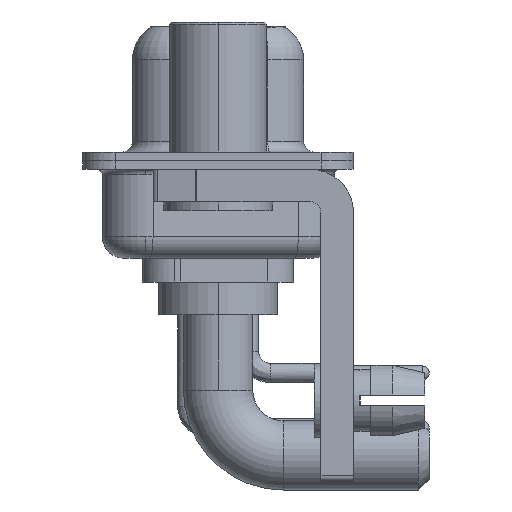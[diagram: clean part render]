
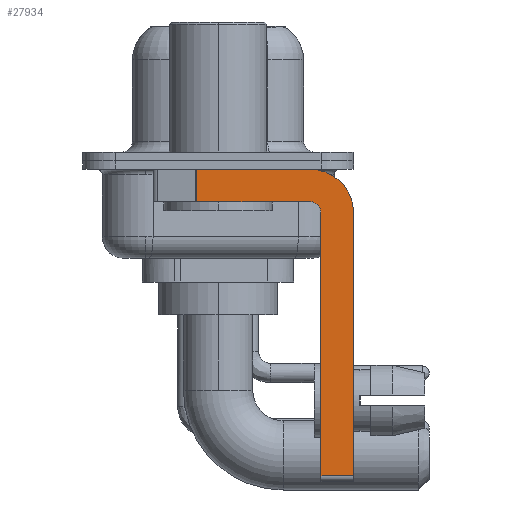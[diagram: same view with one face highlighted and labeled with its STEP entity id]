
A CAD part, left-side view. The second image highlights one B-rep face of the part: STEP entity #27934.
In plain terms, the highlighted planar face has unit normal (-1, 0, 0).
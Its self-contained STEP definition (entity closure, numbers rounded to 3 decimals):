
#461 = CARTESIAN_POINT ( 'NONE',  ( -2.9, -4.75, -14.55 ) ) ;
#1003 = VECTOR ( 'NONE', #2084, 1000. ) ;
#1038 = DIRECTION ( 'NONE',  ( 1., 0., 0. ) ) ;
#1607 = DIRECTION ( 'NONE',  ( 0., 0., -1. ) ) ;
#2084 = DIRECTION ( 'NONE',  ( 0., 1., 0. ) ) ;
#2692 = EDGE_CURVE ( 'NONE', #20505, #5850, #7778, .T. ) ;
#3034 = EDGE_CURVE ( 'NONE', #7729, #13837, #23552, .T. ) ;
#3617 = DIRECTION ( 'NONE',  ( 0., -1., 0. ) ) ;
#4566 = EDGE_CURVE ( 'NONE', #24103, #5850, #14656, .T. ) ;
#4975 = CARTESIAN_POINT ( 'NONE',  ( -2.9, -4.25, -2.4 ) ) ;
#5219 = ORIENTED_EDGE ( 'NONE', *, *, #21026, .F. ) ;
#5723 = ORIENTED_EDGE ( 'NONE', *, *, #12915, .F. ) ;
#5760 = DIRECTION ( 'NONE',  ( 0., 0., -1. ) ) ;
#5808 = ORIENTED_EDGE ( 'NONE', *, *, #2692, .T. ) ;
#5850 = VERTEX_POINT ( 'NONE', #18707 ) ;
#5950 = EDGE_CURVE ( 'NONE', #20505, #19403, #23986, .T. ) ;
#6567 = VECTOR ( 'NONE', #3617, 1000. ) ;
#7017 = VECTOR ( 'NONE', #5760, 1000. ) ;
#7421 = DIRECTION ( 'NONE',  ( 1., 0., 0. ) ) ;
#7729 = VERTEX_POINT ( 'NONE', #27818 ) ;
#7732 = CARTESIAN_POINT ( 'NONE',  ( -2.9, -4.25, -2.4 ) ) ;
#7778 = LINE ( 'NONE', #25280, #6567 ) ;
#8604 = CARTESIAN_POINT ( 'NONE',  ( -2.9, -4.75, -2.4 ) ) ;
#8954 = AXIS2_PLACEMENT_3D ( 'NONE', #7732, #25233, #12316 ) ;
#9681 = AXIS2_PLACEMENT_3D ( 'NONE', #4975, #7421, #21334 ) ;
#9824 = CARTESIAN_POINT ( 'NONE',  ( -2.9, -4.25, -0.4 ) ) ;
#10072 = LINE ( 'NONE', #12357, #25252 ) ;
#10833 = CARTESIAN_POINT ( 'NONE',  ( -2.9, -4.25, -1.9 ) ) ;
#10846 = CARTESIAN_POINT ( 'NONE',  ( -2.9, -6.25, -2.4 ) ) ;
#12316 = DIRECTION ( 'NONE',  ( 0., 0., 1. ) ) ;
#12357 = CARTESIAN_POINT ( 'NONE',  ( -2.9, 3., -0.4 ) ) ;
#12915 = EDGE_CURVE ( 'NONE', #7729, #17468, #10072, .T. ) ;
#13186 = ORIENTED_EDGE ( 'NONE', *, *, #4566, .F. ) ;
#13837 = VERTEX_POINT ( 'NONE', #26151 ) ;
#13858 = ORIENTED_EDGE ( 'NONE', *, *, #14041, .F. ) ;
#14041 = EDGE_CURVE ( 'NONE', #17468, #24103, #20267, .T. ) ;
#14102 = DIRECTION ( 'NONE',  ( 0., 0., -1. ) ) ;
#14165 = VERTEX_POINT ( 'NONE', #16093 ) ;
#14656 = LINE ( 'NONE', #21135, #22841 ) ;
#14734 = ORIENTED_EDGE ( 'NONE', *, *, #28105, .F. ) ;
#14936 = CARTESIAN_POINT ( 'NONE',  ( -2.9, -4.75, -14.8 ) ) ;
#14976 = EDGE_LOOP ( 'NONE', ( #5723, #15237, #14734, #5219, #22424, #5808, #13186, #13858 ) ) ;
#15237 = ORIENTED_EDGE ( 'NONE', *, *, #3034, .T. ) ;
#15307 = CARTESIAN_POINT ( 'NONE',  ( -2.9, 0.978, -1.9 ) ) ;
#16093 = CARTESIAN_POINT ( 'NONE',  ( -2.9, -4.25, -1.9 ) ) ;
#17468 = VERTEX_POINT ( 'NONE', #9824 ) ;
#17906 = PLANE ( 'NONE',  #9681 ) ;
#18707 = CARTESIAN_POINT ( 'NONE',  ( -2.9, -6.25, -14.55 ) ) ;
#18967 = VECTOR ( 'NONE', #23704, 1000. ) ;
#19403 = VERTEX_POINT ( 'NONE', #8604 ) ;
#20267 = CIRCLE ( 'NONE', #24837, 2. ) ;
#20428 = CARTESIAN_POINT ( 'NONE',  ( -2.9, -4.25, -2.4 ) ) ;
#20505 = VERTEX_POINT ( 'NONE', #461 ) ;
#21026 = EDGE_CURVE ( 'NONE', #19403, #14165, #21331, .T. ) ;
#21120 = DIRECTION ( 'NONE',  ( 0., -1., 0. ) ) ;
#21135 = CARTESIAN_POINT ( 'NONE',  ( -2.9, -6.25, -2.4 ) ) ;
#21331 = CIRCLE ( 'NONE', #8954, 0.5 ) ;
#21334 = DIRECTION ( 'NONE',  ( 0., 0., -1. ) ) ;
#21610 = LINE ( 'NONE', #10833, #1003 ) ;
#22424 = ORIENTED_EDGE ( 'NONE', *, *, #5950, .F. ) ;
#22841 = VECTOR ( 'NONE', #1607, 1000. ) ;
#23552 = LINE ( 'NONE', #15307, #7017 ) ;
#23704 = DIRECTION ( 'NONE',  ( 0., 0., 1. ) ) ;
#23986 = LINE ( 'NONE', #14936, #18967 ) ;
#24103 = VERTEX_POINT ( 'NONE', #10846 ) ;
#24837 = AXIS2_PLACEMENT_3D ( 'NONE', #20428, #1038, #14102 ) ;
#25233 = DIRECTION ( 'NONE',  ( -1., 0., 0. ) ) ;
#25252 = VECTOR ( 'NONE', #21120, 1000. ) ;
#25280 = CARTESIAN_POINT ( 'NONE',  ( -2.9, -4.25, -14.55 ) ) ;
#26151 = CARTESIAN_POINT ( 'NONE',  ( -2.9, 0.978, -1.9 ) ) ;
#27077 = FACE_OUTER_BOUND ( 'NONE', #14976, .T. ) ;
#27818 = CARTESIAN_POINT ( 'NONE',  ( -2.9, 0.978, -0.4 ) ) ;
#27934 = ADVANCED_FACE ( 'NONE', ( #27077 ), #17906, .F. ) ;
#28105 = EDGE_CURVE ( 'NONE', #14165, #13837, #21610, .T. ) ;
